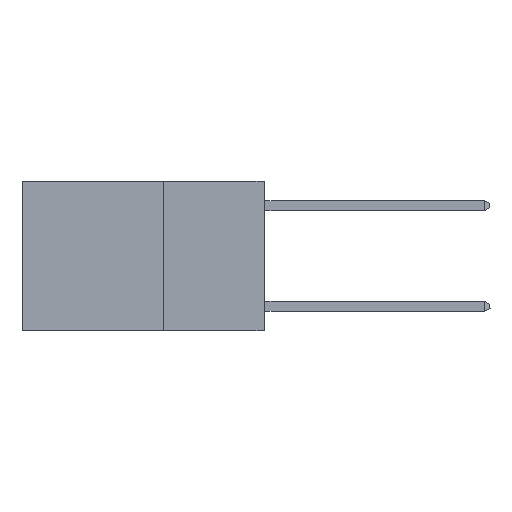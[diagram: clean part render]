
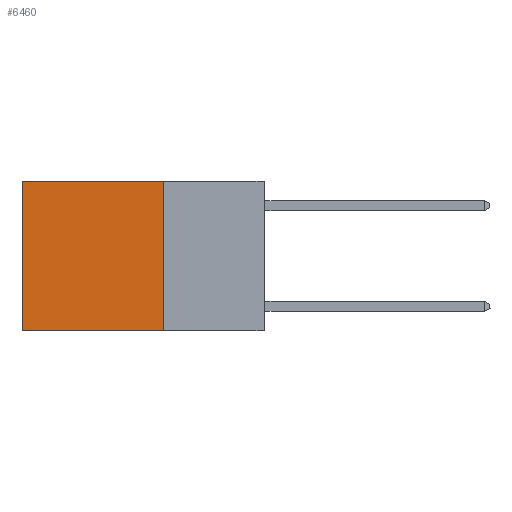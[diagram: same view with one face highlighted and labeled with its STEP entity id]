
A CAD part, left-side view. The second image highlights one B-rep face of the part: STEP entity #6460.
In plain terms, the highlighted planar face has unit normal (-1, 0, 0).
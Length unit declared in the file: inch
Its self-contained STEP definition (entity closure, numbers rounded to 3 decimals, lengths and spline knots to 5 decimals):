
#305 = LINE ( 'NONE', #6272, #6537 ) ;
#563 = ORIENTED_EDGE ( 'NONE', *, *, #4170, .T. ) ;
#1055 = LINE ( 'NONE', #5021, #8681 ) ;
#1312 = VECTOR ( 'NONE', #1744, 39.37008 ) ;
#1511 = CARTESIAN_POINT ( 'NONE',  ( 0.2625, 0.25, 0. ) ) ;
#1627 = CARTESIAN_POINT ( 'NONE',  ( 0.2625, 0.25, -0.37 ) ) ;
#1744 = DIRECTION ( 'NONE',  ( 0., 0., -1. ) ) ;
#1846 = VECTOR ( 'NONE', #8447, 39.37008 ) ;
#2816 = EDGE_CURVE ( 'NONE', #3161, #2918, #1055, .T. ) ;
#2918 = VERTEX_POINT ( 'NONE', #9057 ) ;
#3161 = VERTEX_POINT ( 'NONE', #1511 ) ;
#3427 = DIRECTION ( 'NONE',  ( 0., 1., 0. ) ) ;
#3438 = CARTESIAN_POINT ( 'NONE',  ( 0.2625, 0.6, 0. ) ) ;
#3903 = EDGE_CURVE ( 'NONE', #3161, #6241, #5682, .T. ) ;
#3911 = DIRECTION ( 'NONE',  ( 1., 0., 0. ) ) ;
#4170 = EDGE_CURVE ( 'NONE', #2918, #4304, #9600, .T. ) ;
#4304 = VERTEX_POINT ( 'NONE', #6654 ) ;
#5021 = CARTESIAN_POINT ( 'NONE',  ( 0.2625, 0.25, 0. ) ) ;
#5082 = AXIS2_PLACEMENT_3D ( 'NONE', #9498, #3911, #7140 ) ;
#5207 = FACE_OUTER_BOUND ( 'NONE', #5444, .T. ) ;
#5444 = EDGE_LOOP ( 'NONE', ( #563, #8257, #5980, #8723 ) ) ;
#5473 = DIRECTION ( 'NONE',  ( 0., 1., 0. ) ) ;
#5682 = LINE ( 'NONE', #8077, #1846 ) ;
#5980 = ORIENTED_EDGE ( 'NONE', *, *, #3903, .F. ) ;
#6210 = PLANE ( 'NONE',  #5082 ) ;
#6241 = VERTEX_POINT ( 'NONE', #1627 ) ;
#6272 = CARTESIAN_POINT ( 'NONE',  ( 0.2625, 0.25, -0.37 ) ) ;
#6460 = ADVANCED_FACE ( 'NONE', ( #5207 ), #6210, .F. ) ;
#6537 = VECTOR ( 'NONE', #5473, 39.37008 ) ;
#6654 = CARTESIAN_POINT ( 'NONE',  ( 0.2625, 0.6, -0.37 ) ) ;
#7140 = DIRECTION ( 'NONE',  ( 0., 0., -1. ) ) ;
#7743 = EDGE_CURVE ( 'NONE', #6241, #4304, #305, .T. ) ;
#8077 = CARTESIAN_POINT ( 'NONE',  ( 0.2625, 0.25, 0. ) ) ;
#8257 = ORIENTED_EDGE ( 'NONE', *, *, #7743, .F. ) ;
#8447 = DIRECTION ( 'NONE',  ( 0., 0., -1. ) ) ;
#8681 = VECTOR ( 'NONE', #3427, 39.37008 ) ;
#8723 = ORIENTED_EDGE ( 'NONE', *, *, #2816, .T. ) ;
#9057 = CARTESIAN_POINT ( 'NONE',  ( 0.2625, 0.6, 0. ) ) ;
#9498 = CARTESIAN_POINT ( 'NONE',  ( 0.2625, 0.25, 0. ) ) ;
#9600 = LINE ( 'NONE', #3438, #1312 ) ;
